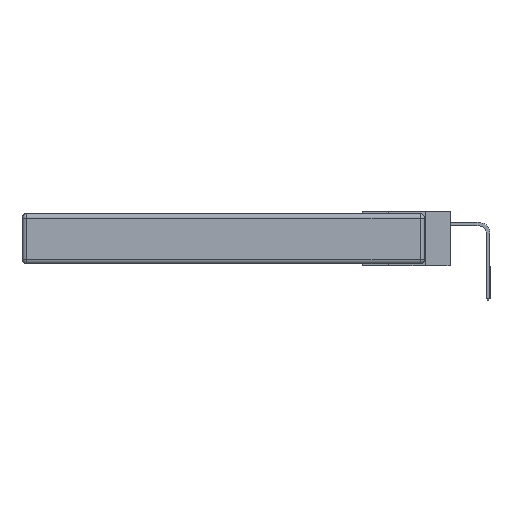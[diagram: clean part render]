
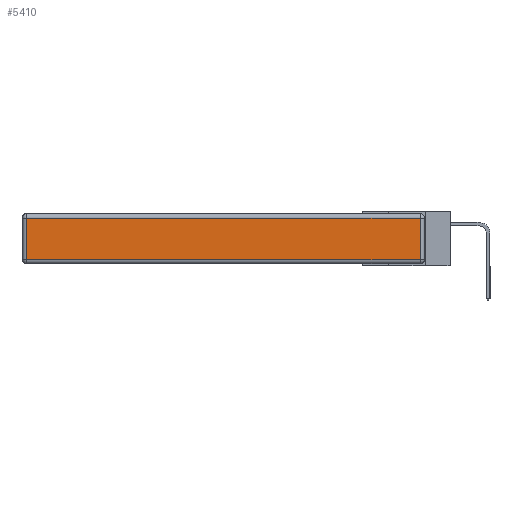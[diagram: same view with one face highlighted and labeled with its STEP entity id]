
A CAD part, left-side view. The second image highlights one B-rep face of the part: STEP entity #5410.
In plain terms, the highlighted planar face has unit normal (-1, 0, 0).
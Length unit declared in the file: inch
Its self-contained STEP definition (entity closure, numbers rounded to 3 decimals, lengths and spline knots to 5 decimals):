
#740 = VERTEX_POINT ( 'NONE', #15168 ) ;
#803 = DIRECTION ( 'NONE',  ( -1., 0., 0. ) ) ;
#2296 = LINE ( 'NONE', #9023, #23532 ) ;
#3465 = ORIENTED_EDGE ( 'NONE', *, *, #14609, .T. ) ;
#5410 = ADVANCED_FACE ( 'NONE', ( #9543 ), #20894, .T. ) ;
#5694 = CARTESIAN_POINT ( 'NONE',  ( 0., 2.72, -0.03 ) ) ;
#5768 = LINE ( 'NONE', #7195, #7194 ) ;
#6548 = EDGE_LOOP ( 'NONE', ( #3465, #8100, #7923, #7470 ) ) ;
#7194 = VECTOR ( 'NONE', #19842, 39.37008 ) ;
#7195 = CARTESIAN_POINT ( 'NONE',  ( 0., 0.03, -0.343 ) ) ;
#7470 = ORIENTED_EDGE ( 'NONE', *, *, #14551, .T. ) ;
#7923 = ORIENTED_EDGE ( 'NONE', *, *, #18742, .T. ) ;
#8100 = ORIENTED_EDGE ( 'NONE', *, *, #14503, .T. ) ;
#8940 = CARTESIAN_POINT ( 'NONE',  ( 0., 0., -0.313 ) ) ;
#9023 = CARTESIAN_POINT ( 'NONE',  ( 0., 2.72, -0.343 ) ) ;
#9543 = FACE_OUTER_BOUND ( 'NONE', #6548, .T. ) ;
#10955 = CARTESIAN_POINT ( 'NONE',  ( 0., 0.03, -0.313 ) ) ;
#10956 = VECTOR ( 'NONE', #12449, 39.37008 ) ;
#11761 = VERTEX_POINT ( 'NONE', #16324 ) ;
#11821 = CARTESIAN_POINT ( 'NONE',  ( 0., 0., -0.343 ) ) ;
#12442 = VERTEX_POINT ( 'NONE', #10955 ) ;
#12449 = DIRECTION ( 'NONE',  ( 0., -1., 0. ) ) ;
#14325 = CARTESIAN_POINT ( 'NONE',  ( 0., 2.75, -0.03 ) ) ;
#14503 = EDGE_CURVE ( 'NONE', #12442, #11761, #5768, .T. ) ;
#14551 = EDGE_CURVE ( 'NONE', #18229, #740, #2296, .T. ) ;
#14609 = EDGE_CURVE ( 'NONE', #740, #12442, #15520, .T. ) ;
#15168 = CARTESIAN_POINT ( 'NONE',  ( 0., 2.72, -0.313 ) ) ;
#15520 = LINE ( 'NONE', #8940, #10956 ) ;
#16324 = CARTESIAN_POINT ( 'NONE',  ( 0., 0.03, -0.03 ) ) ;
#17907 = DIRECTION ( 'NONE',  ( 0., 0., 1. ) ) ;
#18084 = LINE ( 'NONE', #14325, #23008 ) ;
#18229 = VERTEX_POINT ( 'NONE', #5694 ) ;
#18742 = EDGE_CURVE ( 'NONE', #11761, #18229, #18084, .T. ) ;
#18760 = AXIS2_PLACEMENT_3D ( 'NONE', #11821, #803, #17907 ) ;
#19842 = DIRECTION ( 'NONE',  ( 0., 0., 1. ) ) ;
#20894 = PLANE ( 'NONE',  #18760 ) ;
#21764 = DIRECTION ( 'NONE',  ( 0., 0., -1. ) ) ;
#23008 = VECTOR ( 'NONE', #23266, 39.37008 ) ;
#23266 = DIRECTION ( 'NONE',  ( 0., 1., 0. ) ) ;
#23532 = VECTOR ( 'NONE', #21764, 39.37008 ) ;
